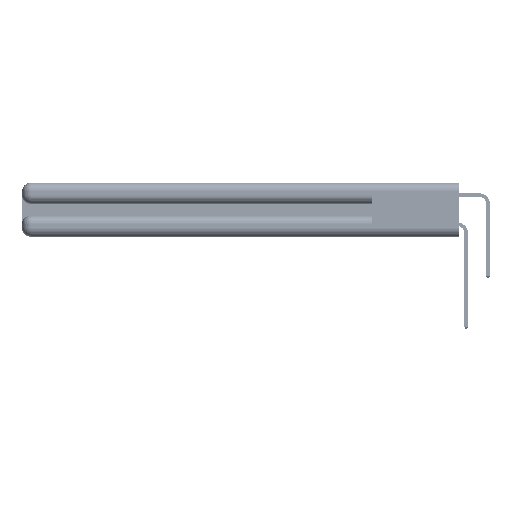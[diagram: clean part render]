
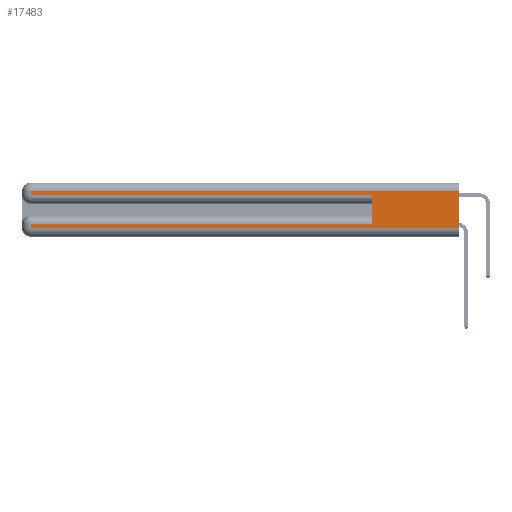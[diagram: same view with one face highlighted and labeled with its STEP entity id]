
A CAD part, left-side view. The second image highlights one B-rep face of the part: STEP entity #17483.
In plain terms, the highlighted planar face has unit normal (-1, 0, 0).
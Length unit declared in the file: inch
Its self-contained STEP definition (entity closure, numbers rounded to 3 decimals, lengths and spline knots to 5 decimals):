
#600 = VECTOR ( 'NONE', #18322, 39.37008 ) ;
#925 = VERTEX_POINT ( 'NONE', #15537 ) ;
#1579 = VECTOR ( 'NONE', #41387, 39.37008 ) ;
#3961 = ORIENTED_EDGE ( 'NONE', *, *, #24027, .T. ) ;
#5512 = EDGE_CURVE ( 'NONE', #16290, #21597, #31616, .T. ) ;
#6241 = DIRECTION ( 'NONE',  ( 0., -1., 0. ) ) ;
#6781 = EDGE_LOOP ( 'NONE', ( #19880, #53500, #23863, #3961, #17867, #40401, #52867, #13258 ) ) ;
#6800 = LINE ( 'NONE', #52298, #47807 ) ;
#7087 = VERTEX_POINT ( 'NONE', #53535 ) ;
#7105 = CARTESIAN_POINT ( 'NONE',  ( 0., 0., 0.37 ) ) ;
#7534 = CARTESIAN_POINT ( 'NONE',  ( 0., 0., 0.37 ) ) ;
#9489 = CARTESIAN_POINT ( 'NONE',  ( 0., 0., 0.06 ) ) ;
#10388 = VECTOR ( 'NONE', #48223, 39.37008 ) ;
#12486 = VERTEX_POINT ( 'NONE', #51140 ) ;
#13258 = ORIENTED_EDGE ( 'NONE', *, *, #5512, .T. ) ;
#13894 = CARTESIAN_POINT ( 'NONE',  ( 0., 0., 0.31 ) ) ;
#14388 = CARTESIAN_POINT ( 'NONE',  ( 0., 0., 0.06 ) ) ;
#15537 = CARTESIAN_POINT ( 'NONE',  ( 0., 2.94, 0.31 ) ) ;
#15595 = PLANE ( 'NONE',  #17989 ) ;
#16251 = VERTEX_POINT ( 'NONE', #54092 ) ;
#16290 = VERTEX_POINT ( 'NONE', #42005 ) ;
#17483 = ADVANCED_FACE ( 'NONE', ( #24883 ), #15595, .F. ) ;
#17544 = VECTOR ( 'NONE', #6241, 39.37008 ) ;
#17867 = ORIENTED_EDGE ( 'NONE', *, *, #44544, .F. ) ;
#17989 = AXIS2_PLACEMENT_3D ( 'NONE', #7105, #45199, #19892 ) ;
#18154 = DIRECTION ( 'NONE',  ( 0., 1., 0. ) ) ;
#18322 = DIRECTION ( 'NONE',  ( 0., 0., 1. ) ) ;
#19470 = LINE ( 'NONE', #13894, #50485 ) ;
#19880 = ORIENTED_EDGE ( 'NONE', *, *, #24241, .F. ) ;
#19892 = DIRECTION ( 'NONE',  ( 0., 0., -1. ) ) ;
#21057 = DIRECTION ( 'NONE',  ( 0., 0., -1. ) ) ;
#21597 = VERTEX_POINT ( 'NONE', #9489 ) ;
#21703 = VECTOR ( 'NONE', #33234, 39.37008 ) ;
#21880 = LINE ( 'NONE', #43638, #600 ) ;
#23863 = ORIENTED_EDGE ( 'NONE', *, *, #34063, .T. ) ;
#24027 = EDGE_CURVE ( 'NONE', #41779, #16251, #47323, .T. ) ;
#24241 = EDGE_CURVE ( 'NONE', #12486, #21597, #35448, .T. ) ;
#24883 = FACE_OUTER_BOUND ( 'NONE', #6781, .T. ) ;
#31155 = DIRECTION ( 'NONE',  ( 0., 1., 0. ) ) ;
#31469 = CARTESIAN_POINT ( 'NONE',  ( 0., 2.94, 0.085 ) ) ;
#31616 = LINE ( 'NONE', #14388, #10388 ) ;
#31631 = CARTESIAN_POINT ( 'NONE',  ( 0., 0., 0.285 ) ) ;
#32616 = VERTEX_POINT ( 'NONE', #31469 ) ;
#33234 = DIRECTION ( 'NONE',  ( 0., 0., -1. ) ) ;
#34063 = EDGE_CURVE ( 'NONE', #925, #41779, #54005, .T. ) ;
#35448 = LINE ( 'NONE', #7534, #1579 ) ;
#35839 = VECTOR ( 'NONE', #21057, 39.37008 ) ;
#40401 = ORIENTED_EDGE ( 'NONE', *, *, #50317, .T. ) ;
#41387 = DIRECTION ( 'NONE',  ( 0., 0., -1. ) ) ;
#41779 = VERTEX_POINT ( 'NONE', #48824 ) ;
#42005 = CARTESIAN_POINT ( 'NONE',  ( 0., 2.94, 0.06 ) ) ;
#42122 = CARTESIAN_POINT ( 'NONE',  ( 0., 2.94, 0.37 ) ) ;
#43638 = CARTESIAN_POINT ( 'NONE',  ( 0., 0.6, 0.145 ) ) ;
#44544 = EDGE_CURVE ( 'NONE', #7087, #16251, #21880, .T. ) ;
#45199 = DIRECTION ( 'NONE',  ( 1., 0., 0. ) ) ;
#47323 = LINE ( 'NONE', #31631, #17544 ) ;
#47807 = VECTOR ( 'NONE', #31155, 39.37008 ) ;
#48223 = DIRECTION ( 'NONE',  ( 0., -1., 0. ) ) ;
#48321 = LINE ( 'NONE', #42122, #35839 ) ;
#48824 = CARTESIAN_POINT ( 'NONE',  ( 0., 2.94, 0.285 ) ) ;
#50155 = CARTESIAN_POINT ( 'NONE',  ( 0., 2.94, 0.37 ) ) ;
#50317 = EDGE_CURVE ( 'NONE', #7087, #32616, #6800, .T. ) ;
#50485 = VECTOR ( 'NONE', #18154, 39.37008 ) ;
#51140 = CARTESIAN_POINT ( 'NONE',  ( 0., 0., 0.31 ) ) ;
#51398 = EDGE_CURVE ( 'NONE', #32616, #16290, #48321, .T. ) ;
#52298 = CARTESIAN_POINT ( 'NONE',  ( 0., 0., 0.085 ) ) ;
#52867 = ORIENTED_EDGE ( 'NONE', *, *, #51398, .T. ) ;
#53036 = EDGE_CURVE ( 'NONE', #12486, #925, #19470, .T. ) ;
#53500 = ORIENTED_EDGE ( 'NONE', *, *, #53036, .T. ) ;
#53535 = CARTESIAN_POINT ( 'NONE',  ( 0., 0.6, 0.085 ) ) ;
#54005 = LINE ( 'NONE', #50155, #21703 ) ;
#54092 = CARTESIAN_POINT ( 'NONE',  ( 0., 0.6, 0.285 ) ) ;
